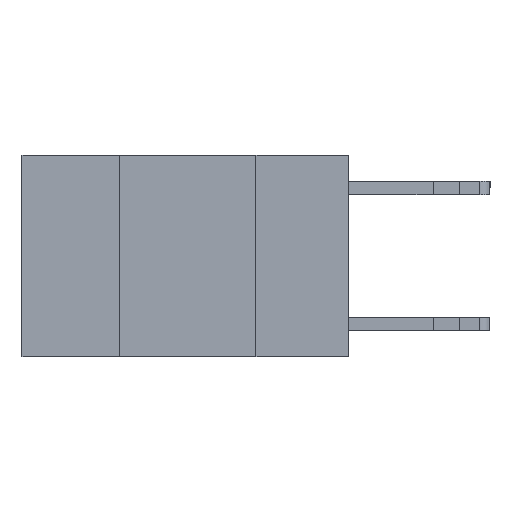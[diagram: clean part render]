
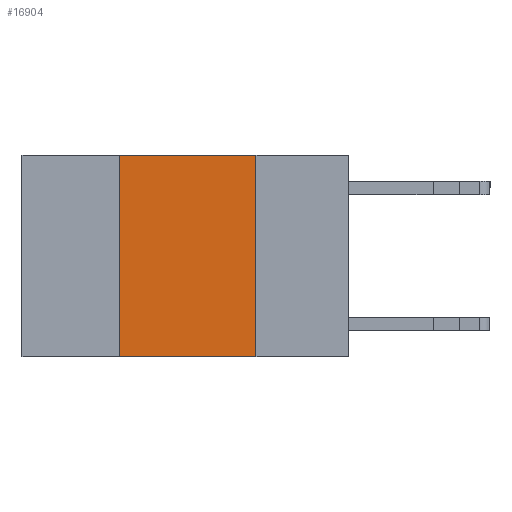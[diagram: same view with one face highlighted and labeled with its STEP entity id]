
A CAD part, left-side view. The second image highlights one B-rep face of the part: STEP entity #16904.
In plain terms, the highlighted planar face has unit normal (-1, 0, 0).
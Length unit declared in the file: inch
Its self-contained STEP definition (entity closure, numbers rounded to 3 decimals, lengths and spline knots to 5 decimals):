
#499 = EDGE_LOOP ( 'NONE', ( #1892, #11110, #2468, #7111 ) ) ;
#556 = CARTESIAN_POINT ( 'NONE',  ( 0., 0.6, -0.37 ) ) ;
#888 = FACE_OUTER_BOUND ( 'NONE', #499, .T. ) ;
#1184 = AXIS2_PLACEMENT_3D ( 'NONE', #9219, #6491, #16777 ) ;
#1259 = CARTESIAN_POINT ( 'NONE',  ( 0., 0.42, 0. ) ) ;
#1575 = CARTESIAN_POINT ( 'NONE',  ( 0., 0.17, -0.37 ) ) ;
#1892 = ORIENTED_EDGE ( 'NONE', *, *, #14555, .F. ) ;
#2468 = ORIENTED_EDGE ( 'NONE', *, *, #7717, .F. ) ;
#2839 = VERTEX_POINT ( 'NONE', #9475 ) ;
#3776 = DIRECTION ( 'NONE',  ( 0., -1., 0. ) ) ;
#5043 = VECTOR ( 'NONE', #14250, 39.37008 ) ;
#5050 = PLANE ( 'NONE',  #1184 ) ;
#5482 = CARTESIAN_POINT ( 'NONE',  ( 0., 0.17, 0. ) ) ;
#6235 = CARTESIAN_POINT ( 'NONE',  ( 0., 0.17, 0. ) ) ;
#6294 = VERTEX_POINT ( 'NONE', #12611 ) ;
#6491 = DIRECTION ( 'NONE',  ( 1., 0., 0. ) ) ;
#7111 = ORIENTED_EDGE ( 'NONE', *, *, #10163, .T. ) ;
#7561 = VECTOR ( 'NONE', #9074, 39.37008 ) ;
#7717 = EDGE_CURVE ( 'NONE', #6294, #2839, #12991, .T. ) ;
#9074 = DIRECTION ( 'NONE',  ( 0., 0., -1. ) ) ;
#9219 = CARTESIAN_POINT ( 'NONE',  ( 0., 0.6, 0. ) ) ;
#9475 = CARTESIAN_POINT ( 'NONE',  ( 0., 0.42, 0. ) ) ;
#9766 = EDGE_CURVE ( 'NONE', #2839, #10204, #18346, .T. ) ;
#10163 = EDGE_CURVE ( 'NONE', #6294, #18140, #10579, .T. ) ;
#10204 = VERTEX_POINT ( 'NONE', #5482 ) ;
#10579 = LINE ( 'NONE', #556, #14409 ) ;
#11110 = ORIENTED_EDGE ( 'NONE', *, *, #9766, .F. ) ;
#12575 = DIRECTION ( 'NONE',  ( 0., -1., 0. ) ) ;
#12611 = CARTESIAN_POINT ( 'NONE',  ( 0., 0.42, -0.37 ) ) ;
#12991 = LINE ( 'NONE', #1259, #5043 ) ;
#14250 = DIRECTION ( 'NONE',  ( 0., 0., 1. ) ) ;
#14409 = VECTOR ( 'NONE', #12575, 39.37008 ) ;
#14555 = EDGE_CURVE ( 'NONE', #10204, #18140, #17855, .T. ) ;
#16777 = DIRECTION ( 'NONE',  ( 0., 0., -1. ) ) ;
#16904 = ADVANCED_FACE ( 'NONE', ( #888 ), #5050, .F. ) ;
#17695 = VECTOR ( 'NONE', #3776, 39.37008 ) ;
#17855 = LINE ( 'NONE', #6235, #7561 ) ;
#18140 = VERTEX_POINT ( 'NONE', #1575 ) ;
#18176 = CARTESIAN_POINT ( 'NONE',  ( 0., 0.6, 0. ) ) ;
#18346 = LINE ( 'NONE', #18176, #17695 ) ;
